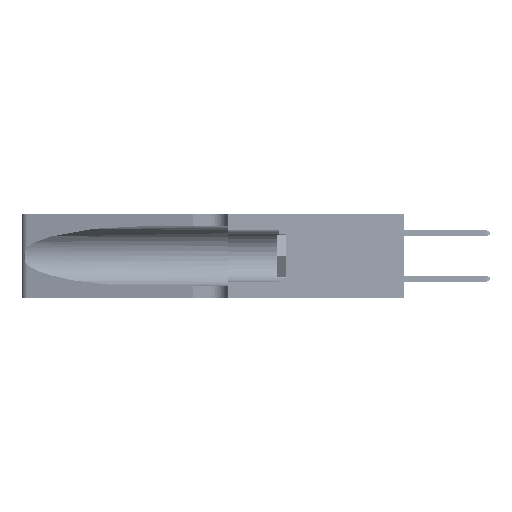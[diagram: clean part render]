
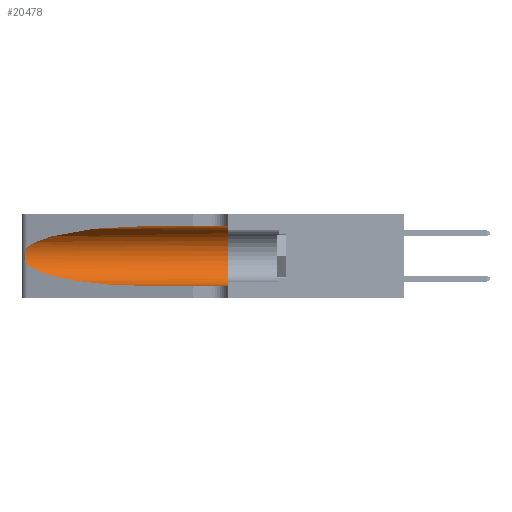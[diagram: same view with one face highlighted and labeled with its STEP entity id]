
A CAD part, left-side view. The second image highlights one B-rep face of the part: STEP entity #20478.
In plain terms, the highlighted cylindrical face has radius 3.308 mm (diameter 6.617 mm), a partial arc.
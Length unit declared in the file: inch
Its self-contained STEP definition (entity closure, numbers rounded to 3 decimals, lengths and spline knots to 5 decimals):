
#279 = CARTESIAN_POINT ( 'NONE',  ( 0.1305, 0.35, 0.185 ) ) ;
#617 = EDGE_CURVE ( 'NONE', #46747, #38247, #39517, .T. ) ;
#875 = CARTESIAN_POINT ( 'NONE',  ( 0.25487, 1.22718, 0.22369 ) ) ;
#1791 = EDGE_CURVE ( 'NONE', #38247, #44512, #27433, .T. ) ;
#5031 = CARTESIAN_POINT ( 'NONE',  ( 0.1305, 0.35, 0.31525 ) ) ;
#5032 = DIRECTION ( 'NONE',  ( 0., 1., 0. ) ) ;
#5481 = CARTESIAN_POINT ( 'NONE',  ( 0.1305, 0.72297, 0.31525 ) ) ;
#5675 = EDGE_CURVE ( 'NONE', #46747, #39636, #14784, .T. ) ;
#7474 = CARTESIAN_POINT ( 'NONE',  ( 0.25487, 1.22718, 0.22369 ) ) ;
#7651 = CARTESIAN_POINT ( 'NONE',  ( 0.25487, 1.22718, 0.14631 ) ) ;
#8116 = EDGE_CURVE ( 'NONE', #9407, #44512, #49791, .T. ) ;
#9407 = VERTEX_POINT ( 'NONE', #47040 ) ;
#10382 = CYLINDRICAL_SURFACE ( 'NONE', #38621, 0.13025 ) ;
#10478 = CARTESIAN_POINT ( 'NONE',  ( 0.2373, 1.15595, 0.28018 ) ) ;
#12278 = CARTESIAN_POINT ( 'NONE',  ( 0.1305, 0.72297, 0.05475 ) ) ;
#13473 = DIRECTION ( 'NONE',  ( 0., -1., 0. ) ) ;
#14784 =( BOUNDED_CURVE ( )  B_SPLINE_CURVE ( 3, ( #27281, #31581, #10478, #43643 ),
 .UNSPECIFIED., .F., .F. ) 
 B_SPLINE_CURVE_WITH_KNOTS ( ( 4, 4 ),
 ( 1.5708, 2.84003 ),
 .UNSPECIFIED. ) 
 CURVE ( )  GEOMETRIC_REPRESENTATION_ITEM ( )  RATIONAL_B_SPLINE_CURVE ( ( 1., 0.87, 0.87, 1. ) ) 
 REPRESENTATION_ITEM ( '' )  );
#15978 = CARTESIAN_POINT ( 'NONE',  ( 0.25789, 1.23486, 0.15765 ) ) ;
#16325 = CARTESIAN_POINT ( 'NONE',  ( 0.25854, 1.2359, 0.20912 ) ) ;
#16723 = CARTESIAN_POINT ( 'NONE',  ( 0.25487, 1.22718, 0.14631 ) ) ;
#17510 = VERTEX_POINT ( 'NONE', #52192 ) ;
#17536 = ORIENTED_EDGE ( 'NONE', *, *, #8116, .T. ) ;
#17553 = CARTESIAN_POINT ( 'NONE',  ( 0.1305, 1.61858, 0.31525 ) ) ;
#19548 = EDGE_CURVE ( 'NONE', #39636, #17510, #46728, .T. ) ;
#20478 = ADVANCED_FACE ( 'NONE', ( #35586 ), #10382, .F. ) ;
#20620 = CARTESIAN_POINT ( 'NONE',  ( 0.25787, 1.23484, 0.2124 ) ) ;
#22978 =( BOUNDED_CURVE ( )  B_SPLINE_CURVE ( 3, ( #16723, #42666, #29859, #12278 ),
 .UNSPECIFIED., .F., .F. ) 
 B_SPLINE_CURVE_WITH_KNOTS ( ( 4, 4 ),
 ( 3.44316, 4.71239 ),
 .UNSPECIFIED. ) 
 CURVE ( )  GEOMETRIC_REPRESENTATION_ITEM ( )  RATIONAL_B_SPLINE_CURVE ( ( 1., 0.87, 0.87, 1. ) ) 
 REPRESENTATION_ITEM ( '' )  );
#24315 = CARTESIAN_POINT ( 'NONE',  ( 0.25555, 1.22994, 0.2215 ) ) ;
#25762 = DIRECTION ( 'NONE',  ( 0., 0., 1. ) ) ;
#26059 = CARTESIAN_POINT ( 'NONE',  ( 0.1305, 1.61858, 0.185 ) ) ;
#26142 = DIRECTION ( 'NONE',  ( 0., -1., 0. ) ) ;
#27281 = CARTESIAN_POINT ( 'NONE',  ( 0.1305, 0.72297, 0.31525 ) ) ;
#27433 = CIRCLE ( 'NONE', #54356, 0.13025 ) ;
#28549 = CARTESIAN_POINT ( 'NONE',  ( 0.26017, 1.23833, 0.17102 ) ) ;
#29100 = CARTESIAN_POINT ( 'NONE',  ( 0.25639, 1.23184, 0.21858 ) ) ;
#29859 = CARTESIAN_POINT ( 'NONE',  ( 0.18966, 0.96281, 0.05475 ) ) ;
#29877 = ORIENTED_EDGE ( 'NONE', *, *, #5675, .T. ) ;
#31581 = CARTESIAN_POINT ( 'NONE',  ( 0.18966, 0.96281, 0.31525 ) ) ;
#33012 = CARTESIAN_POINT ( 'NONE',  ( 0.26018, 1.23835, 0.19895 ) ) ;
#33040 = EDGE_LOOP ( 'NONE', ( #29877, #35986, #47720, #17536, #52126, #49054 ) ) ;
#33208 = VECTOR ( 'NONE', #26142, 39.37008 ) ;
#33693 = DIRECTION ( 'NONE',  ( 0., -1., 0. ) ) ;
#33824 = EDGE_CURVE ( 'NONE', #17510, #9407, #22978, .T. ) ;
#34515 = CARTESIAN_POINT ( 'NONE',  ( 0.1305, 1.61858, 0.05475 ) ) ;
#35586 = FACE_OUTER_BOUND ( 'NONE', #33040, .T. ) ;
#35986 = ORIENTED_EDGE ( 'NONE', *, *, #19548, .T. ) ;
#37112 = CARTESIAN_POINT ( 'NONE',  ( 0.25856, 1.23593, 0.16098 ) ) ;
#37560 = CARTESIAN_POINT ( 'NONE',  ( 0.1305, 0.35, 0.05475 ) ) ;
#38247 = VERTEX_POINT ( 'NONE', #5031 ) ;
#38621 = AXIS2_PLACEMENT_3D ( 'NONE', #26059, #13473, #42389 ) ;
#39517 = LINE ( 'NONE', #17553, #43533 ) ;
#39636 = VERTEX_POINT ( 'NONE', #875 ) ;
#41513 = CARTESIAN_POINT ( 'NONE',  ( 0.26075, 1.23896, 0.178 ) ) ;
#41713 = CARTESIAN_POINT ( 'NONE',  ( 0.25555, 1.22993, 0.14849 ) ) ;
#42389 = DIRECTION ( 'NONE',  ( 0., 0., -1. ) ) ;
#42666 = CARTESIAN_POINT ( 'NONE',  ( 0.2373, 1.15595, 0.08982 ) ) ;
#43533 = VECTOR ( 'NONE', #33693, 39.37008 ) ;
#43643 = CARTESIAN_POINT ( 'NONE',  ( 0.25487, 1.22718, 0.22369 ) ) ;
#44512 = VERTEX_POINT ( 'NONE', #37560 ) ;
#46728 = B_SPLINE_CURVE_WITH_KNOTS ( 'NONE', 3,
 ( #7474, #24315, #29100, #20620, #16325, #33012, #49862, #41513, #28549, #37112, #15978, #54309, #41713, #7651 ),
 .UNSPECIFIED., .F., .F.,
 ( 4, 2, 2, 2, 2, 2, 4 ),
 ( 0., 0.00027, 0.00053, 0.00107, 0.0016, 0.00187, 0.00214 ),
 .UNSPECIFIED. ) ;
#46747 = VERTEX_POINT ( 'NONE', #5481 ) ;
#47040 = CARTESIAN_POINT ( 'NONE',  ( 0.1305, 0.72297, 0.05475 ) ) ;
#47720 = ORIENTED_EDGE ( 'NONE', *, *, #33824, .T. ) ;
#49054 = ORIENTED_EDGE ( 'NONE', *, *, #617, .F. ) ;
#49791 = LINE ( 'NONE', #34515, #33208 ) ;
#49862 = CARTESIAN_POINT ( 'NONE',  ( 0.26075, 1.23896, 0.19203 ) ) ;
#52126 = ORIENTED_EDGE ( 'NONE', *, *, #1791, .F. ) ;
#52192 = CARTESIAN_POINT ( 'NONE',  ( 0.25487, 1.22718, 0.14631 ) ) ;
#54309 = CARTESIAN_POINT ( 'NONE',  ( 0.25639, 1.23186, 0.15144 ) ) ;
#54356 = AXIS2_PLACEMENT_3D ( 'NONE', #279, #5032, #25762 ) ;
